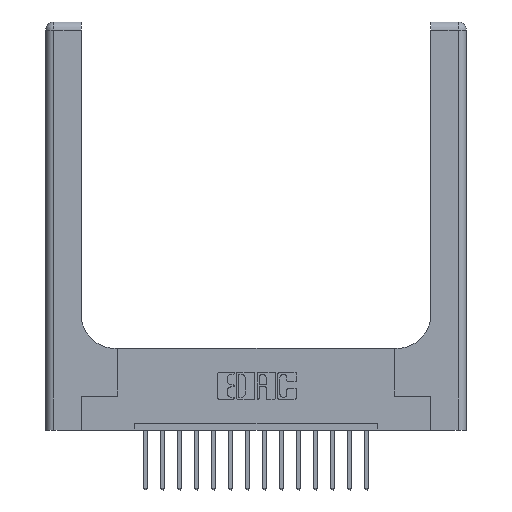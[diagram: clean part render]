
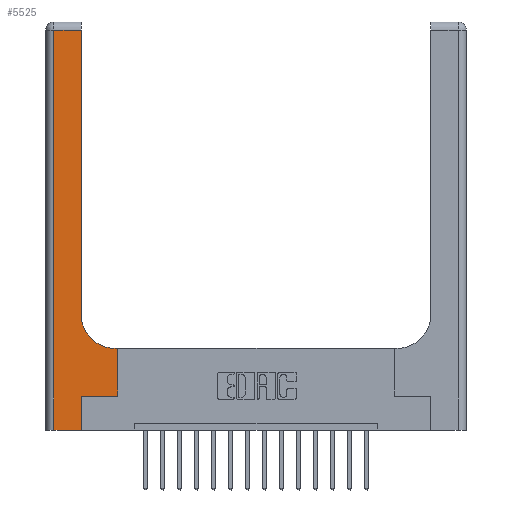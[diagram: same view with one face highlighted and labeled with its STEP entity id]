
A CAD part, top view. The second image highlights one B-rep face of the part: STEP entity #5525.
In plain terms, the highlighted planar face has unit normal (0, 0, 1).
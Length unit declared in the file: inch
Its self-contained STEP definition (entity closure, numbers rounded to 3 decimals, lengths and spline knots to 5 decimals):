
#227 = CARTESIAN_POINT ( 'NONE',  ( 0.06, 3., 0.37 ) ) ;
#681 = CARTESIAN_POINT ( 'NONE',  ( 0.26, 0.6, 0.37 ) ) ;
#982 = EDGE_CURVE ( 'NONE', #12326, #7889, #5543, .T. ) ;
#986 = EDGE_CURVE ( 'NONE', #15726, #14630, #9748, .T. ) ;
#1007 = VECTOR ( 'NONE', #15983, 39.37008 ) ;
#1012 = CARTESIAN_POINT ( 'NONE',  ( 0.528, 0.25, 0.37 ) ) ;
#1226 = EDGE_CURVE ( 'NONE', #5432, #8698, #12048, .T. ) ;
#1343 = ORIENTED_EDGE ( 'NONE', *, *, #12694, .T. ) ;
#1448 = CARTESIAN_POINT ( 'NONE',  ( 0.51, 0.85, 0.37 ) ) ;
#1588 = EDGE_CURVE ( 'NONE', #8698, #12326, #2508, .T. ) ;
#1647 = VECTOR ( 'NONE', #16302, 39.37008 ) ;
#1966 = CARTESIAN_POINT ( 'NONE',  ( 0., 0., 0.37 ) ) ;
#2236 = VECTOR ( 'NONE', #17071, 39.37008 ) ;
#2307 = VECTOR ( 'NONE', #4355, 39.37008 ) ;
#2508 = CIRCLE ( 'NONE', #16823, 0.25 ) ;
#2674 = VECTOR ( 'NONE', #17072, 39.37008 ) ;
#2868 = ORIENTED_EDGE ( 'NONE', *, *, #1226, .T. ) ;
#4002 = DIRECTION ( 'NONE',  ( 0., 1., 0. ) ) ;
#4105 = ORIENTED_EDGE ( 'NONE', *, *, #986, .T. ) ;
#4355 = DIRECTION ( 'NONE',  ( 0., 1., 0. ) ) ;
#4415 = VERTEX_POINT ( 'NONE', #9357 ) ;
#4794 = ORIENTED_EDGE ( 'NONE', *, *, #12689, .T. ) ;
#4843 = VERTEX_POINT ( 'NONE', #12068 ) ;
#5418 = EDGE_LOOP ( 'NONE', ( #16558, #16856, #4105, #17943, #1343, #4794, #14664, #2868, #8230 ) ) ;
#5432 = VERTEX_POINT ( 'NONE', #11913 ) ;
#5525 = ADVANCED_FACE ( 'NONE', ( #10630 ), #9250, .F. ) ;
#5543 = LINE ( 'NONE', #16533, #10422 ) ;
#5565 = EDGE_CURVE ( 'NONE', #4415, #5432, #10893, .T. ) ;
#5797 = CARTESIAN_POINT ( 'NONE',  ( 0.265, 0., 0.37 ) ) ;
#7805 = EDGE_CURVE ( 'NONE', #7889, #15726, #15713, .T. ) ;
#7889 = VERTEX_POINT ( 'NONE', #15895 ) ;
#8230 = ORIENTED_EDGE ( 'NONE', *, *, #1588, .T. ) ;
#8433 = CARTESIAN_POINT ( 'NONE',  ( 0.265, 0., 0.37 ) ) ;
#8698 = VERTEX_POINT ( 'NONE', #8801 ) ;
#8801 = CARTESIAN_POINT ( 'NONE',  ( 0.51, 0.6, 0.37 ) ) ;
#9250 = PLANE ( 'NONE',  #10121 ) ;
#9357 = CARTESIAN_POINT ( 'NONE',  ( 0.528, 0.25, 0.37 ) ) ;
#9636 = DIRECTION ( 'NONE',  ( 1., 0., 0. ) ) ;
#9653 = CARTESIAN_POINT ( 'NONE',  ( 0.26, 0.85, 0.37 ) ) ;
#9748 = LINE ( 'NONE', #227, #2236 ) ;
#9869 = DIRECTION ( 'NONE',  ( 1., 0., 0. ) ) ;
#10121 = AXIS2_PLACEMENT_3D ( 'NONE', #17655, #16390, #15088 ) ;
#10422 = VECTOR ( 'NONE', #4002, 39.37008 ) ;
#10498 = VECTOR ( 'NONE', #9636, 39.37008 ) ;
#10630 = FACE_OUTER_BOUND ( 'NONE', #5418, .T. ) ;
#10683 = CARTESIAN_POINT ( 'NONE',  ( 0.06, 2.94, 0.37 ) ) ;
#10893 = LINE ( 'NONE', #1012, #1647 ) ;
#11142 = EDGE_CURVE ( 'NONE', #14630, #17638, #14393, .T. ) ;
#11369 = CARTESIAN_POINT ( 'NONE',  ( 0.06, 0., 0.37 ) ) ;
#11913 = CARTESIAN_POINT ( 'NONE',  ( 0.528, 0.6, 0.37 ) ) ;
#12048 = LINE ( 'NONE', #681, #14198 ) ;
#12068 = CARTESIAN_POINT ( 'NONE',  ( 0.265, 0.25, 0.37 ) ) ;
#12326 = VERTEX_POINT ( 'NONE', #9653 ) ;
#12689 = EDGE_CURVE ( 'NONE', #4843, #4415, #13919, .T. ) ;
#12694 = EDGE_CURVE ( 'NONE', #17638, #4843, #17964, .T. ) ;
#13735 = CARTESIAN_POINT ( 'NONE',  ( 0.265, 0.25, 0.37 ) ) ;
#13919 = LINE ( 'NONE', #13735, #10498 ) ;
#14198 = VECTOR ( 'NONE', #14761, 39.37008 ) ;
#14393 = LINE ( 'NONE', #1966, #2674 ) ;
#14630 = VERTEX_POINT ( 'NONE', #11369 ) ;
#14664 = ORIENTED_EDGE ( 'NONE', *, *, #5565, .T. ) ;
#14761 = DIRECTION ( 'NONE',  ( -1., 0., 0. ) ) ;
#15088 = DIRECTION ( 'NONE',  ( -1., 0., 0. ) ) ;
#15713 = LINE ( 'NONE', #17256, #1007 ) ;
#15726 = VERTEX_POINT ( 'NONE', #10683 ) ;
#15895 = CARTESIAN_POINT ( 'NONE',  ( 0.26, 2.94, 0.37 ) ) ;
#15983 = DIRECTION ( 'NONE',  ( -1., 0., 0. ) ) ;
#16302 = DIRECTION ( 'NONE',  ( 0., 1., 0. ) ) ;
#16390 = DIRECTION ( 'NONE',  ( 0., 0., -1. ) ) ;
#16533 = CARTESIAN_POINT ( 'NONE',  ( 0.26, 3., 0.37 ) ) ;
#16558 = ORIENTED_EDGE ( 'NONE', *, *, #982, .T. ) ;
#16823 = AXIS2_PLACEMENT_3D ( 'NONE', #1448, #17000, #9869 ) ;
#16856 = ORIENTED_EDGE ( 'NONE', *, *, #7805, .T. ) ;
#17000 = DIRECTION ( 'NONE',  ( 0., 0., -1. ) ) ;
#17071 = DIRECTION ( 'NONE',  ( 0., -1., 0. ) ) ;
#17072 = DIRECTION ( 'NONE',  ( 1., 0., 0. ) ) ;
#17256 = CARTESIAN_POINT ( 'NONE',  ( 0., 2.94, 0.37 ) ) ;
#17638 = VERTEX_POINT ( 'NONE', #8433 ) ;
#17655 = CARTESIAN_POINT ( 'NONE',  ( 0., 3., 0.37 ) ) ;
#17943 = ORIENTED_EDGE ( 'NONE', *, *, #11142, .T. ) ;
#17964 = LINE ( 'NONE', #5797, #2307 ) ;
